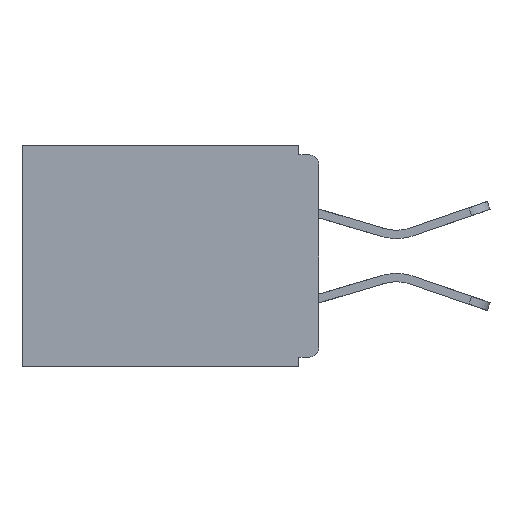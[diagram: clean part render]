
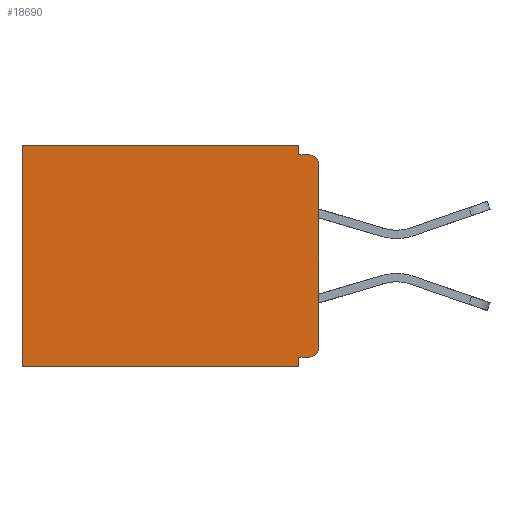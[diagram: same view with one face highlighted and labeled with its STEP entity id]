
A CAD part, left-side view. The second image highlights one B-rep face of the part: STEP entity #18690.
In plain terms, the highlighted planar face has unit normal (-1, 0, 0).
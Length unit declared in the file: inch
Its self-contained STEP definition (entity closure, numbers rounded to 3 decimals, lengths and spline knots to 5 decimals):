
#322 = LINE ( 'NONE', #4554, #7631 ) ;
#472 = CARTESIAN_POINT ( 'NONE',  ( 0.298, 0., 0. ) ) ;
#660 = VECTOR ( 'NONE', #20754, 39.37008 ) ;
#1031 = LINE ( 'NONE', #17669, #14656 ) ;
#1237 = EDGE_CURVE ( 'NONE', #15020, #2779, #20057, .T. ) ;
#1519 = CARTESIAN_POINT ( 'NONE',  ( 0.298, 0., -0.03 ) ) ;
#1877 = VERTEX_POINT ( 'NONE', #9531 ) ;
#1955 = DIRECTION ( 'NONE',  ( 0., 0., -1. ) ) ;
#2217 = ORIENTED_EDGE ( 'NONE', *, *, #16595, .T. ) ;
#2380 = ORIENTED_EDGE ( 'NONE', *, *, #16311, .F. ) ;
#2452 = AXIS2_PLACEMENT_3D ( 'NONE', #20110, #13732, #20176 ) ;
#2505 = DIRECTION ( 'NONE',  ( -1., 0., 0. ) ) ;
#2779 = VERTEX_POINT ( 'NONE', #10822 ) ;
#3163 = AXIS2_PLACEMENT_3D ( 'NONE', #15174, #20225, #12001 ) ;
#3555 = ORIENTED_EDGE ( 'NONE', *, *, #8759, .T. ) ;
#3588 = CARTESIAN_POINT ( 'NONE',  ( 0.298, 0.031, 0. ) ) ;
#3936 = CARTESIAN_POINT ( 'NONE',  ( 0.298, 0.015, -0.015 ) ) ;
#4182 = LINE ( 'NONE', #20187, #13534 ) ;
#4554 = CARTESIAN_POINT ( 'NONE',  ( 0.298, 0., -0.343 ) ) ;
#4630 = CARTESIAN_POINT ( 'NONE',  ( 0.298, 0.031, -0.015 ) ) ;
#5168 = CARTESIAN_POINT ( 'NONE',  ( 0.298, 0., -0.313 ) ) ;
#5714 = LINE ( 'NONE', #472, #11750 ) ;
#6484 = VECTOR ( 'NONE', #7936, 39.37008 ) ;
#7209 = CARTESIAN_POINT ( 'NONE',  ( 0.298, 0.015, -0.313 ) ) ;
#7351 = PLANE ( 'NONE',  #3163 ) ;
#7631 = VECTOR ( 'NONE', #17240, 39.37008 ) ;
#7809 = CARTESIAN_POINT ( 'NONE',  ( 0.298, 0., 0. ) ) ;
#7817 = CARTESIAN_POINT ( 'NONE',  ( 0.298, 0.031, -0.343 ) ) ;
#7936 = DIRECTION ( 'NONE',  ( 0., 0., -1. ) ) ;
#8085 = AXIS2_PLACEMENT_3D ( 'NONE', #7209, #2505, #18674 ) ;
#8229 = EDGE_CURVE ( 'NONE', #14371, #17421, #14606, .T. ) ;
#8254 = VERTEX_POINT ( 'NONE', #17288 ) ;
#8759 = EDGE_CURVE ( 'NONE', #1877, #20533, #17599, .T. ) ;
#9531 = CARTESIAN_POINT ( 'NONE',  ( 0.298, 0.015, -0.328 ) ) ;
#9567 = VECTOR ( 'NONE', #13866, 39.37008 ) ;
#9724 = EDGE_CURVE ( 'NONE', #13846, #11756, #17808, .T. ) ;
#10160 = CARTESIAN_POINT ( 'NONE',  ( 0.298, 0.031, -0.343 ) ) ;
#10219 = CARTESIAN_POINT ( 'NONE',  ( 0.298, 0.031, -0.328 ) ) ;
#10367 = CARTESIAN_POINT ( 'NONE',  ( 0.298, 0.46, 0. ) ) ;
#10580 = VERTEX_POINT ( 'NONE', #14604 ) ;
#10822 = CARTESIAN_POINT ( 'NONE',  ( 0.298, 0.031, -0.343 ) ) ;
#11482 = VECTOR ( 'NONE', #1955, 39.37008 ) ;
#11685 = EDGE_CURVE ( 'NONE', #2779, #10580, #322, .T. ) ;
#11750 = VECTOR ( 'NONE', #19855, 39.37008 ) ;
#11756 = VERTEX_POINT ( 'NONE', #4630 ) ;
#12001 = DIRECTION ( 'NONE',  ( 0., 0., -1. ) ) ;
#12895 = ORIENTED_EDGE ( 'NONE', *, *, #14210, .F. ) ;
#13509 = ORIENTED_EDGE ( 'NONE', *, *, #9724, .F. ) ;
#13534 = VECTOR ( 'NONE', #19988, 39.37008 ) ;
#13732 = DIRECTION ( 'NONE',  ( -1., 0., 0. ) ) ;
#13846 = VERTEX_POINT ( 'NONE', #3588 ) ;
#13866 = DIRECTION ( 'NONE',  ( 0., 0., -1. ) ) ;
#13917 = LINE ( 'NONE', #10367, #9567 ) ;
#14086 = ORIENTED_EDGE ( 'NONE', *, *, #1237, .F. ) ;
#14210 = EDGE_CURVE ( 'NONE', #11756, #17421, #1031, .T. ) ;
#14252 = ORIENTED_EDGE ( 'NONE', *, *, #8229, .T. ) ;
#14371 = VERTEX_POINT ( 'NONE', #1519 ) ;
#14455 = EDGE_CURVE ( 'NONE', #8254, #10580, #13917, .T. ) ;
#14604 = CARTESIAN_POINT ( 'NONE',  ( 0.298, 0.46, -0.343 ) ) ;
#14606 = CIRCLE ( 'NONE', #2452, 0.015 ) ;
#14656 = VECTOR ( 'NONE', #19302, 39.37008 ) ;
#15020 = VERTEX_POINT ( 'NONE', #10219 ) ;
#15174 = CARTESIAN_POINT ( 'NONE',  ( 0.298, 0., 0. ) ) ;
#15333 = ORIENTED_EDGE ( 'NONE', *, *, #14455, .T. ) ;
#15954 = ORIENTED_EDGE ( 'NONE', *, *, #16649, .F. ) ;
#16043 = LINE ( 'NONE', #7809, #6484 ) ;
#16311 = EDGE_CURVE ( 'NONE', #14371, #20533, #16043, .T. ) ;
#16595 = EDGE_CURVE ( 'NONE', #13846, #8254, #5714, .T. ) ;
#16649 = EDGE_CURVE ( 'NONE', #1877, #15020, #4182, .T. ) ;
#16723 = FACE_OUTER_BOUND ( 'NONE', #19731, .T. ) ;
#17240 = DIRECTION ( 'NONE',  ( 0., 1., 0. ) ) ;
#17288 = CARTESIAN_POINT ( 'NONE',  ( 0.298, 0.46, 0. ) ) ;
#17421 = VERTEX_POINT ( 'NONE', #3936 ) ;
#17599 = CIRCLE ( 'NONE', #8085, 0.015 ) ;
#17669 = CARTESIAN_POINT ( 'NONE',  ( 0.298, 0., -0.015 ) ) ;
#17808 = LINE ( 'NONE', #7817, #660 ) ;
#18178 = ORIENTED_EDGE ( 'NONE', *, *, #11685, .F. ) ;
#18674 = DIRECTION ( 'NONE',  ( 0., 0., -1. ) ) ;
#18690 = ADVANCED_FACE ( 'NONE', ( #16723 ), #7351, .F. ) ;
#19302 = DIRECTION ( 'NONE',  ( 0., -1., 0. ) ) ;
#19731 = EDGE_LOOP ( 'NONE', ( #14252, #12895, #13509, #2217, #15333, #18178, #14086, #15954, #3555, #2380 ) ) ;
#19855 = DIRECTION ( 'NONE',  ( 0., 1., 0. ) ) ;
#19988 = DIRECTION ( 'NONE',  ( 0., 1., 0. ) ) ;
#20057 = LINE ( 'NONE', #10160, #11482 ) ;
#20110 = CARTESIAN_POINT ( 'NONE',  ( 0.298, 0.015, -0.03 ) ) ;
#20176 = DIRECTION ( 'NONE',  ( 0., 0., -1. ) ) ;
#20187 = CARTESIAN_POINT ( 'NONE',  ( 0.298, 0., -0.328 ) ) ;
#20225 = DIRECTION ( 'NONE',  ( 1., 0., 0. ) ) ;
#20533 = VERTEX_POINT ( 'NONE', #5168 ) ;
#20754 = DIRECTION ( 'NONE',  ( 0., 0., -1. ) ) ;
